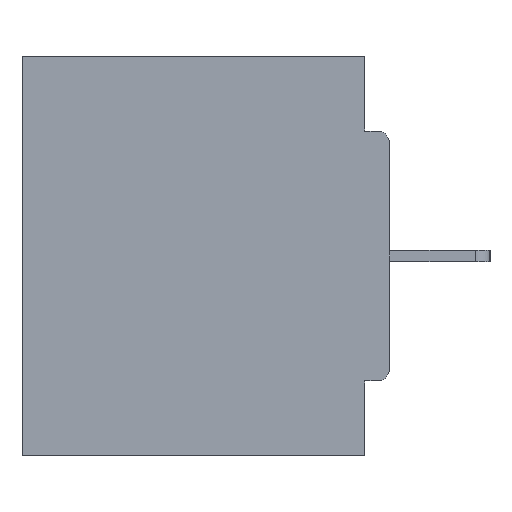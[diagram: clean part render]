
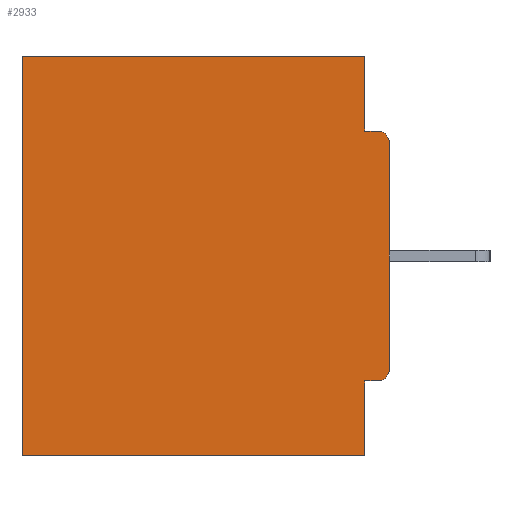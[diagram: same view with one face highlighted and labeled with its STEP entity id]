
A CAD part, left-side view. The second image highlights one B-rep face of the part: STEP entity #2933.
In plain terms, the highlighted planar face has unit normal (-1, 0, 0).
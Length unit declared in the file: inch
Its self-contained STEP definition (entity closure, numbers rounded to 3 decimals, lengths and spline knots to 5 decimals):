
#115 = DIRECTION ( 'NONE',  ( 0., 1., 0. ) ) ;
#938 = DIRECTION ( 'NONE',  ( 0., 0., -1. ) ) ;
#1174 = LINE ( 'NONE', #11441, #12712 ) ;
#1176 = CARTESIAN_POINT ( 'NONE',  ( 0.298, 0.031, -0.0935 ) ) ;
#1182 = ORIENTED_EDGE ( 'NONE', *, *, #30773, .F. ) ;
#1390 = CARTESIAN_POINT ( 'NONE',  ( 0.298, 0., 0. ) ) ;
#1446 = DIRECTION ( 'NONE',  ( -1., 0., 0. ) ) ;
#1615 = CARTESIAN_POINT ( 'NONE',  ( 0.298, 0.015, -0.3915 ) ) ;
#1875 = DIRECTION ( 'NONE',  ( 0., 0., -1. ) ) ;
#1975 = ORIENTED_EDGE ( 'NONE', *, *, #25394, .F. ) ;
#2108 = AXIS2_PLACEMENT_3D ( 'NONE', #12429, #2678, #10064 ) ;
#2210 = DIRECTION ( 'NONE',  ( 0., 0., -1. ) ) ;
#2241 = VERTEX_POINT ( 'NONE', #27145 ) ;
#2340 = CARTESIAN_POINT ( 'NONE',  ( 0.298, 0.031, 0. ) ) ;
#2415 = CARTESIAN_POINT ( 'NONE',  ( 0.298, 0.031, -0.4065 ) ) ;
#2651 = EDGE_CURVE ( 'NONE', #22189, #27021, #1174, .T. ) ;
#2678 = DIRECTION ( 'NONE',  ( -1., 0., 0. ) ) ;
#2743 = VERTEX_POINT ( 'NONE', #16460 ) ;
#2933 = ADVANCED_FACE ( 'NONE', ( #23183 ), #25528, .F. ) ;
#3491 = CARTESIAN_POINT ( 'NONE',  ( 0.298, 0., -0.0935 ) ) ;
#3841 = EDGE_CURVE ( 'NONE', #14528, #25621, #5725, .T. ) ;
#4072 = VECTOR ( 'NONE', #20699, 39.37008 ) ;
#4378 = EDGE_CURVE ( 'NONE', #25621, #2241, #29536, .T. ) ;
#4407 = CARTESIAN_POINT ( 'NONE',  ( 0.298, 0.46, 0. ) ) ;
#4613 = EDGE_CURVE ( 'NONE', #14528, #7721, #12564, .T. ) ;
#5102 = VERTEX_POINT ( 'NONE', #23107 ) ;
#5180 = VECTOR ( 'NONE', #6520, 39.37008 ) ;
#5316 = EDGE_CURVE ( 'NONE', #7721, #27021, #29941, .T. ) ;
#5725 = LINE ( 'NONE', #13150, #4072 ) ;
#6520 = DIRECTION ( 'NONE',  ( 0., -1., 0. ) ) ;
#6596 = LINE ( 'NONE', #1390, #19001 ) ;
#6619 = VECTOR ( 'NONE', #29570, 39.37008 ) ;
#6769 = ORIENTED_EDGE ( 'NONE', *, *, #19611, .T. ) ;
#6923 = DIRECTION ( 'NONE',  ( 0., 0., -1. ) ) ;
#7415 = LINE ( 'NONE', #9602, #28311 ) ;
#7721 = VERTEX_POINT ( 'NONE', #9131 ) ;
#9013 = CARTESIAN_POINT ( 'NONE',  ( 0.298, 0., -0.3915 ) ) ;
#9131 = CARTESIAN_POINT ( 'NONE',  ( 0.298, 0.46, 0. ) ) ;
#9602 = CARTESIAN_POINT ( 'NONE',  ( 0.298, 0.031, -0.5 ) ) ;
#9625 = CIRCLE ( 'NONE', #24641, 0.015 ) ;
#9826 = EDGE_CURVE ( 'NONE', #5102, #2241, #16037, .T. ) ;
#10064 = DIRECTION ( 'NONE',  ( 0., 0., -1. ) ) ;
#10573 = DIRECTION ( 'NONE',  ( 0., 0., -1. ) ) ;
#11161 = EDGE_LOOP ( 'NONE', ( #13289, #18054, #28469, #23867, #12761, #29944, #1975, #1182, #6769, #31262 ) ) ;
#11297 = VERTEX_POINT ( 'NONE', #9013 ) ;
#11441 = CARTESIAN_POINT ( 'NONE',  ( 0.298, 0., -0.5 ) ) ;
#12429 = CARTESIAN_POINT ( 'NONE',  ( 0.298, 0.015, -0.1085 ) ) ;
#12564 = LINE ( 'NONE', #12733, #23429 ) ;
#12712 = VECTOR ( 'NONE', #29571, 39.37008 ) ;
#12733 = CARTESIAN_POINT ( 'NONE',  ( 0.298, 0., 0. ) ) ;
#12761 = ORIENTED_EDGE ( 'NONE', *, *, #5316, .T. ) ;
#12892 = VECTOR ( 'NONE', #6923, 39.37008 ) ;
#13082 = CARTESIAN_POINT ( 'NONE',  ( 0.298, 0.46, -0.5 ) ) ;
#13150 = CARTESIAN_POINT ( 'NONE',  ( 0.298, 0.031, -0.5 ) ) ;
#13289 = ORIENTED_EDGE ( 'NONE', *, *, #9826, .T. ) ;
#14528 = VERTEX_POINT ( 'NONE', #2340 ) ;
#16037 = CIRCLE ( 'NONE', #2108, 0.015 ) ;
#16460 = CARTESIAN_POINT ( 'NONE',  ( 0.298, 0.015, -0.4065 ) ) ;
#18054 = ORIENTED_EDGE ( 'NONE', *, *, #4378, .F. ) ;
#18117 = DIRECTION ( 'NONE',  ( 1., 0., 0. ) ) ;
#19001 = VECTOR ( 'NONE', #1875, 39.37008 ) ;
#19311 = LINE ( 'NONE', #19477, #6619 ) ;
#19477 = CARTESIAN_POINT ( 'NONE',  ( 0.298, 0., -0.4065 ) ) ;
#19611 = EDGE_CURVE ( 'NONE', #2743, #11297, #9625, .T. ) ;
#20699 = DIRECTION ( 'NONE',  ( 0., 0., -1. ) ) ;
#22133 = AXIS2_PLACEMENT_3D ( 'NONE', #31240, #18117, #10573 ) ;
#22189 = VERTEX_POINT ( 'NONE', #31758 ) ;
#23107 = CARTESIAN_POINT ( 'NONE',  ( 0.298, 0., -0.1085 ) ) ;
#23183 = FACE_OUTER_BOUND ( 'NONE', #11161, .T. ) ;
#23429 = VECTOR ( 'NONE', #115, 39.37008 ) ;
#23712 = VERTEX_POINT ( 'NONE', #2415 ) ;
#23867 = ORIENTED_EDGE ( 'NONE', *, *, #4613, .T. ) ;
#24641 = AXIS2_PLACEMENT_3D ( 'NONE', #1615, #1446, #938 ) ;
#25394 = EDGE_CURVE ( 'NONE', #23712, #22189, #7415, .T. ) ;
#25528 = PLANE ( 'NONE',  #22133 ) ;
#25621 = VERTEX_POINT ( 'NONE', #1176 ) ;
#27021 = VERTEX_POINT ( 'NONE', #13082 ) ;
#27145 = CARTESIAN_POINT ( 'NONE',  ( 0.298, 0.015, -0.0935 ) ) ;
#28311 = VECTOR ( 'NONE', #2210, 39.37008 ) ;
#28469 = ORIENTED_EDGE ( 'NONE', *, *, #3841, .F. ) ;
#29536 = LINE ( 'NONE', #3491, #5180 ) ;
#29570 = DIRECTION ( 'NONE',  ( 0., 1., 0. ) ) ;
#29571 = DIRECTION ( 'NONE',  ( 0., 1., 0. ) ) ;
#29941 = LINE ( 'NONE', #4407, #12892 ) ;
#29944 = ORIENTED_EDGE ( 'NONE', *, *, #2651, .F. ) ;
#30773 = EDGE_CURVE ( 'NONE', #2743, #23712, #19311, .T. ) ;
#31240 = CARTESIAN_POINT ( 'NONE',  ( 0.298, 0., 0. ) ) ;
#31262 = ORIENTED_EDGE ( 'NONE', *, *, #31542, .F. ) ;
#31542 = EDGE_CURVE ( 'NONE', #5102, #11297, #6596, .T. ) ;
#31758 = CARTESIAN_POINT ( 'NONE',  ( 0.298, 0.031, -0.5 ) ) ;
